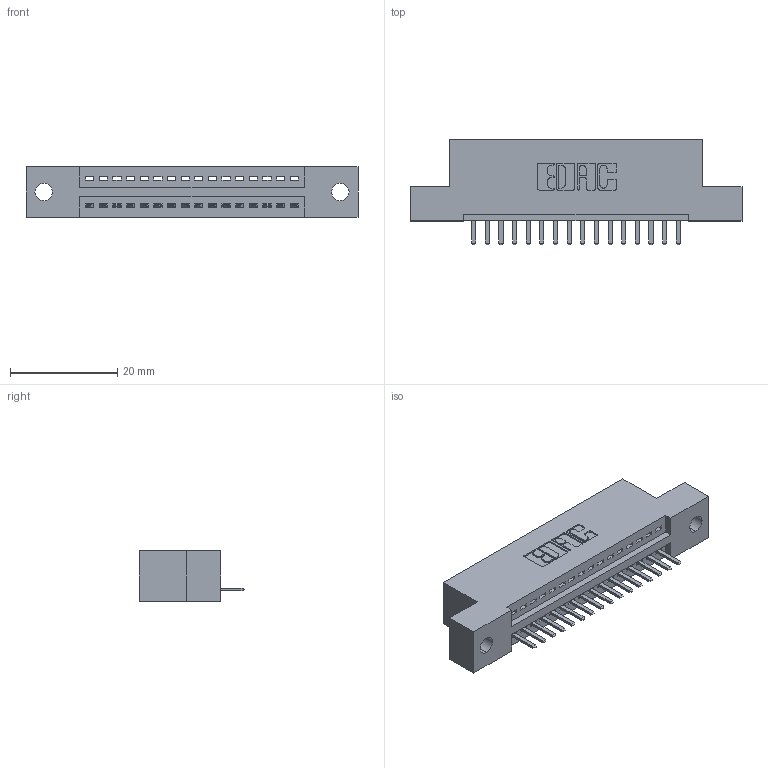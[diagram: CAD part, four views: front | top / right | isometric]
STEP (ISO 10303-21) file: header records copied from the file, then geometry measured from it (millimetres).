
FILE_DESCRIPTION (( 'STEP AP203' ), '1' );
FILE_NAME ('345-016-520-102.STEP', '2019-10-04T13:06:55', ( '' ), ( '' ), 'SwSTEP 2.0', 'SolidWorks 2016', '' );
FILE_SCHEMA (( 'CONFIG_CONTROL_DESIGN' ));
Length unit declared in the file: inch
Products named in the file (3): 345-292-001_345-293-120; 345 Part_Flush Mounting Lugs - 0.128 Dia; 345-016-520-102
Assembly tree (17 placements, depth 2):
  345-016-520-102
    345 Part_Flush Mounting Lugs - 0.128 Dia
    345-292-001_345-293-120  x16
Bounding box: 61.85 x 19.68 x 9.4 mm (x, y, z)
Volume: 5578.8 mm3; surface area: 6638.3 mm2
Topology: 17 solids, 17 shells, 1118 faces, 3285 edges, 2146 vertices
Faces by surface type: plane 752, cylinder 366
Entity records: 15659 total; most frequent: CARTESIAN_POINT 2732, ORIENTED_EDGE 2670, DIRECTION 2411, EDGE_CURVE 1335, VECTOR 1135, LINE 1135, VERTEX_POINT 886, AXIS2_PLACEMENT_3D 638
